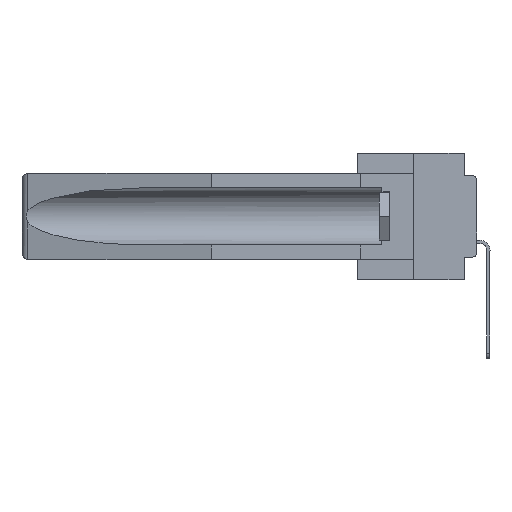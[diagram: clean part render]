
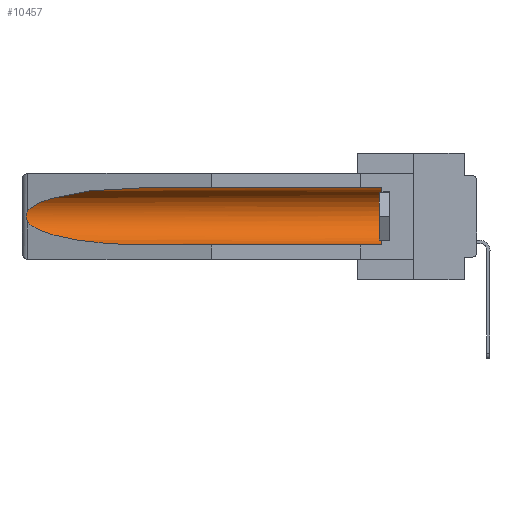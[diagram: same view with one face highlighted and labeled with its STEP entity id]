
A CAD part, left-side view. The second image highlights one B-rep face of the part: STEP entity #10457.
In plain terms, the highlighted cylindrical face has radius 2.857 mm (diameter 5.715 mm), a partial arc.
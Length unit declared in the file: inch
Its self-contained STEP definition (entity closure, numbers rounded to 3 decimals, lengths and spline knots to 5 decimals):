
#476 = CARTESIAN_POINT ( 'NONE',  ( 0.2673, 1.53269, -0.17917 ) ) ;
#478 = VERTEX_POINT ( 'NONE', #12862 ) ;
#1242 = EDGE_LOOP ( 'NONE', ( #7665, #27731, #11857, #6332, #19075, #7400 ) ) ;
#2846 = CARTESIAN_POINT ( 'NONE',  ( 0.26537, 1.52718, -0.19328 ) ) ;
#3370 = VERTEX_POINT ( 'NONE', #14041 ) ;
#5093 = CARTESIAN_POINT ( 'NONE',  ( 0.2675, 1.53308, -0.16763 ) ) ;
#5502 = CARTESIAN_POINT ( 'NONE',  ( 0.26597, 1.5296, -0.19026 ) ) ;
#5635 = VECTOR ( 'NONE', #21498, 39.37008 ) ;
#6332 = ORIENTED_EDGE ( 'NONE', *, *, #13033, .F. ) ;
#6600 = CARTESIAN_POINT ( 'NONE',  ( 0.25451, 1.48313, -0.24835 ) ) ;
#6853 = VERTEX_POINT ( 'NONE', #29551 ) ;
#7133 = CARTESIAN_POINT ( 'NONE',  ( 0.155, -0.30754, -0.059 ) ) ;
#7400 = ORIENTED_EDGE ( 'NONE', *, *, #15808, .T. ) ;
#7665 = ORIENTED_EDGE ( 'NONE', *, *, #28917, .T. ) ;
#8522 = CARTESIAN_POINT ( 'NONE',  ( 0.155, 1.07973, -0.284 ) ) ;
#8956 = LINE ( 'NONE', #18825, #5635 ) ;
#10457 = ADVANCED_FACE ( 'NONE', ( #20008 ), #13788, .F. ) ;
#11375 = DIRECTION ( 'NONE',  ( 0., 1., 0. ) ) ;
#11484 = CARTESIAN_POINT ( 'NONE',  ( 0.21114, 1.30732, -0.284 ) ) ;
#11857 = ORIENTED_EDGE ( 'NONE', *, *, #14046, .T. ) ;
#12054 = VECTOR ( 'NONE', #11375, 39.37008 ) ;
#12199 = CARTESIAN_POINT ( 'NONE',  ( 0.26597, 1.52961, -0.15275 ) ) ;
#12681 =( BOUNDED_CURVE ( )  B_SPLINE_CURVE ( 3, ( #14418, #23985, #19309, #26166 ),
 .UNSPECIFIED., .F., .F. ) 
 B_SPLINE_CURVE_WITH_KNOTS ( ( 4, 4 ),
 ( 4.71239, 6.08839 ),
 .UNSPECIFIED. ) 
 CURVE ( )  GEOMETRIC_REPRESENTATION_ITEM ( )  RATIONAL_B_SPLINE_CURVE ( ( 1., 0.848, 0.848, 1. ) ) 
 REPRESENTATION_ITEM ( '' )  );
#12862 = CARTESIAN_POINT ( 'NONE',  ( 0.155, 1.07973, -0.059 ) ) ;
#13033 = EDGE_CURVE ( 'NONE', #23568, #6853, #8956, .T. ) ;
#13443 = CARTESIAN_POINT ( 'NONE',  ( 0.155, -0.30754, -0.1715 ) ) ;
#13788 = CYLINDRICAL_SURFACE ( 'NONE', #20143, 0.1125 ) ;
#14041 = CARTESIAN_POINT ( 'NONE',  ( 0.155, 0.126, -0.059 ) ) ;
#14046 = EDGE_CURVE ( 'NONE', #17162, #6853, #22262, .T. ) ;
#14418 = CARTESIAN_POINT ( 'NONE',  ( 0.155, 1.07973, -0.059 ) ) ;
#14844 = CIRCLE ( 'NONE', #18892, 0.1125 ) ;
#15804 = VERTEX_POINT ( 'NONE', #25474 ) ;
#15808 = EDGE_CURVE ( 'NONE', #3370, #478, #24977, .T. ) ;
#16115 = CARTESIAN_POINT ( 'NONE',  ( 0.155, 0.126, -0.284 ) ) ;
#17162 = VERTEX_POINT ( 'NONE', #17710 ) ;
#17202 = CARTESIAN_POINT ( 'NONE',  ( 0.2675, 1.53308, -0.17534 ) ) ;
#17710 = CARTESIAN_POINT ( 'NONE',  ( 0.26537, 1.52718, -0.19328 ) ) ;
#17742 = B_SPLINE_CURVE_WITH_KNOTS ( 'NONE', 3,
 ( #19255, #12199, #26495, #28964, #5093, #17202, #476, #28855, #5502, #2846 ),
 .UNSPECIFIED., .F., .F.,
 ( 4, 2, 2, 2, 4 ),
 ( 0., 0.00029, 0.00058, 0.00087, 0.00117 ),
 .UNSPECIFIED. ) ;
#18825 = CARTESIAN_POINT ( 'NONE',  ( 0.155, -0.30754, -0.284 ) ) ;
#18837 = CARTESIAN_POINT ( 'NONE',  ( 0.155, 0.126, -0.1715 ) ) ;
#18892 = AXIS2_PLACEMENT_3D ( 'NONE', #18837, #21307, #30423 ) ;
#19075 = ORIENTED_EDGE ( 'NONE', *, *, #19547, .T. ) ;
#19255 = CARTESIAN_POINT ( 'NONE',  ( 0.26537, 1.52718, -0.14972 ) ) ;
#19309 = CARTESIAN_POINT ( 'NONE',  ( 0.25451, 1.48313, -0.09465 ) ) ;
#19547 = EDGE_CURVE ( 'NONE', #23568, #3370, #14844, .T. ) ;
#20008 = FACE_OUTER_BOUND ( 'NONE', #1242, .T. ) ;
#20143 = AXIS2_PLACEMENT_3D ( 'NONE', #13443, #29706, #28033 ) ;
#20645 = CARTESIAN_POINT ( 'NONE',  ( 0.26537, 1.52718, -0.19328 ) ) ;
#21307 = DIRECTION ( 'NONE',  ( 0., -1., 0. ) ) ;
#21498 = DIRECTION ( 'NONE',  ( 0., 1., 0. ) ) ;
#22262 =( BOUNDED_CURVE ( )  B_SPLINE_CURVE ( 3, ( #20645, #6600, #11484, #8522 ),
 .UNSPECIFIED., .F., .F. ) 
 B_SPLINE_CURVE_WITH_KNOTS ( ( 4, 4 ),
 ( 0.1948, 1.5708 ),
 .UNSPECIFIED. ) 
 CURVE ( )  GEOMETRIC_REPRESENTATION_ITEM ( )  RATIONAL_B_SPLINE_CURVE ( ( 1., 0.848, 0.848, 1. ) ) 
 REPRESENTATION_ITEM ( '' )  );
#23568 = VERTEX_POINT ( 'NONE', #16115 ) ;
#23985 = CARTESIAN_POINT ( 'NONE',  ( 0.21114, 1.30732, -0.059 ) ) ;
#24977 = LINE ( 'NONE', #7133, #12054 ) ;
#25474 = CARTESIAN_POINT ( 'NONE',  ( 0.26537, 1.52718, -0.14972 ) ) ;
#26166 = CARTESIAN_POINT ( 'NONE',  ( 0.26537, 1.52718, -0.14972 ) ) ;
#26495 = CARTESIAN_POINT ( 'NONE',  ( 0.26654, 1.53092, -0.15636 ) ) ;
#26852 = EDGE_CURVE ( 'NONE', #15804, #17162, #17742, .T. ) ;
#27731 = ORIENTED_EDGE ( 'NONE', *, *, #26852, .T. ) ;
#28033 = DIRECTION ( 'NONE',  ( 0., 0., 1. ) ) ;
#28855 = CARTESIAN_POINT ( 'NONE',  ( 0.26655, 1.53094, -0.18657 ) ) ;
#28917 = EDGE_CURVE ( 'NONE', #478, #15804, #12681, .T. ) ;
#28964 = CARTESIAN_POINT ( 'NONE',  ( 0.2673, 1.5327, -0.16383 ) ) ;
#29551 = CARTESIAN_POINT ( 'NONE',  ( 0.155, 1.07973, -0.284 ) ) ;
#29706 = DIRECTION ( 'NONE',  ( 0., 1., 0. ) ) ;
#30423 = DIRECTION ( 'NONE',  ( 0., 0., 1. ) ) ;
